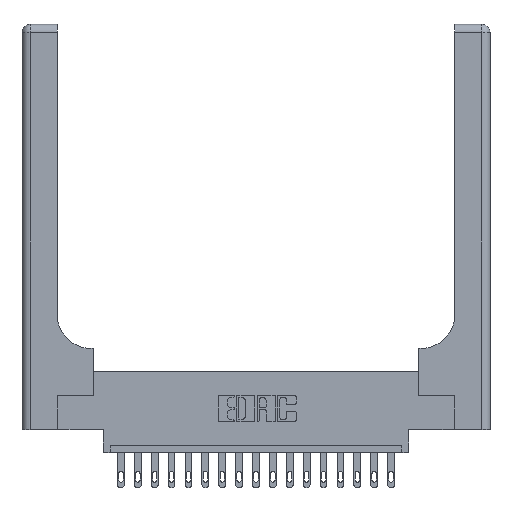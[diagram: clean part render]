
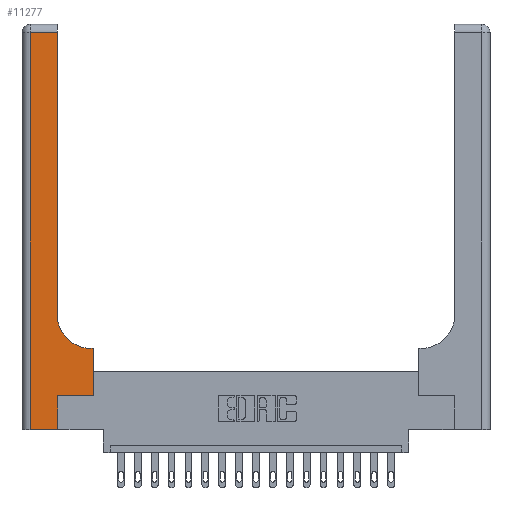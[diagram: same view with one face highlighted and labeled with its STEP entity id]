
A CAD part, top view. The second image highlights one B-rep face of the part: STEP entity #11277.
In plain terms, the highlighted planar face has unit normal (0, 0, 1).
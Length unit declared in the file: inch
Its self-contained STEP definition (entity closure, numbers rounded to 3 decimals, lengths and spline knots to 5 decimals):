
#448 = VERTEX_POINT ( 'NONE', #10915 ) ;
#597 = LINE ( 'NONE', #6665, #10438 ) ;
#862 = DIRECTION ( 'NONE',  ( -1., 0., 0. ) ) ;
#1247 = CARTESIAN_POINT ( 'NONE',  ( 0.26, 2.94, 0.37 ) ) ;
#1666 = VECTOR ( 'NONE', #3041, 39.37008 ) ;
#1766 = VERTEX_POINT ( 'NONE', #1247 ) ;
#1850 = LINE ( 'NONE', #6346, #12595 ) ;
#1892 = EDGE_CURVE ( 'NONE', #11586, #7389, #16539, .T. ) ;
#2382 = CARTESIAN_POINT ( 'NONE',  ( 0.06, 0., 0.37 ) ) ;
#2471 = ORIENTED_EDGE ( 'NONE', *, *, #11147, .T. ) ;
#2693 = DIRECTION ( 'NONE',  ( 0., 1., 0. ) ) ;
#3041 = DIRECTION ( 'NONE',  ( 0., -1., 0. ) ) ;
#3828 = ORIENTED_EDGE ( 'NONE', *, *, #5410, .T. ) ;
#3852 = LINE ( 'NONE', #8823, #18318 ) ;
#3874 = CARTESIAN_POINT ( 'NONE',  ( 0.26, 0.6, 0.37 ) ) ;
#4307 = VERTEX_POINT ( 'NONE', #8676 ) ;
#4693 = DIRECTION ( 'NONE',  ( 0., 1., 0. ) ) ;
#5379 = LINE ( 'NONE', #3874, #12411 ) ;
#5410 = EDGE_CURVE ( 'NONE', #14057, #8418, #8841, .T. ) ;
#5472 = DIRECTION ( 'NONE',  ( -1., 0., 0. ) ) ;
#6346 = CARTESIAN_POINT ( 'NONE',  ( 0.528, 0.25, 0.37 ) ) ;
#6375 = CARTESIAN_POINT ( 'NONE',  ( 0.265, 0., 0.37 ) ) ;
#6446 = CARTESIAN_POINT ( 'NONE',  ( 0.06, 2.94, 0.37 ) ) ;
#6665 = CARTESIAN_POINT ( 'NONE',  ( 0.265, 0.25, 0.37 ) ) ;
#6925 = AXIS2_PLACEMENT_3D ( 'NONE', #7197, #11944, #10188 ) ;
#7197 = CARTESIAN_POINT ( 'NONE',  ( 0.51, 0.85, 0.37 ) ) ;
#7357 = DIRECTION ( 'NONE',  ( 0., 0., -1. ) ) ;
#7389 = VERTEX_POINT ( 'NONE', #2382 ) ;
#7577 = EDGE_CURVE ( 'NONE', #14171, #4307, #1850, .T. ) ;
#8364 = LINE ( 'NONE', #12728, #13408 ) ;
#8418 = VERTEX_POINT ( 'NONE', #10773 ) ;
#8663 = CARTESIAN_POINT ( 'NONE',  ( 0., 3., 0.37 ) ) ;
#8676 = CARTESIAN_POINT ( 'NONE',  ( 0.528, 0.6, 0.37 ) ) ;
#8744 = EDGE_CURVE ( 'NONE', #8418, #1766, #11638, .T. ) ;
#8823 = CARTESIAN_POINT ( 'NONE',  ( 0., 2.94, 0.37 ) ) ;
#8841 = CIRCLE ( 'NONE', #6925, 0.25 ) ;
#9365 = LINE ( 'NONE', #6375, #12979 ) ;
#9778 = ORIENTED_EDGE ( 'NONE', *, *, #15472, .T. ) ;
#9821 = AXIS2_PLACEMENT_3D ( 'NONE', #8663, #7357, #14606 ) ;
#9897 = EDGE_CURVE ( 'NONE', #13454, #14171, #597, .T. ) ;
#10188 = DIRECTION ( 'NONE',  ( 1., 0., 0. ) ) ;
#10438 = VECTOR ( 'NONE', #12729, 39.37008 ) ;
#10483 = ORIENTED_EDGE ( 'NONE', *, *, #10532, .T. ) ;
#10532 = EDGE_CURVE ( 'NONE', #1766, #11586, #3852, .T. ) ;
#10773 = CARTESIAN_POINT ( 'NONE',  ( 0.26, 0.85, 0.37 ) ) ;
#10915 = CARTESIAN_POINT ( 'NONE',  ( 0.265, 0., 0.37 ) ) ;
#11147 = EDGE_CURVE ( 'NONE', #448, #13454, #9365, .T. ) ;
#11277 = ADVANCED_FACE ( 'NONE', ( #13415 ), #19052, .F. ) ;
#11418 = ORIENTED_EDGE ( 'NONE', *, *, #1892, .T. ) ;
#11422 = CARTESIAN_POINT ( 'NONE',  ( 0.51, 0.6, 0.37 ) ) ;
#11586 = VERTEX_POINT ( 'NONE', #6446 ) ;
#11638 = LINE ( 'NONE', #11737, #17058 ) ;
#11737 = CARTESIAN_POINT ( 'NONE',  ( 0.26, 3., 0.37 ) ) ;
#11944 = DIRECTION ( 'NONE',  ( 0., 0., -1. ) ) ;
#12411 = VECTOR ( 'NONE', #5472, 39.37008 ) ;
#12487 = ORIENTED_EDGE ( 'NONE', *, *, #14084, .T. ) ;
#12595 = VECTOR ( 'NONE', #17246, 39.37008 ) ;
#12680 = ORIENTED_EDGE ( 'NONE', *, *, #7577, .T. ) ;
#12728 = CARTESIAN_POINT ( 'NONE',  ( 0., 0., 0.37 ) ) ;
#12729 = DIRECTION ( 'NONE',  ( 1., 0., 0. ) ) ;
#12842 = ORIENTED_EDGE ( 'NONE', *, *, #8744, .T. ) ;
#12979 = VECTOR ( 'NONE', #4693, 39.37008 ) ;
#13112 = CARTESIAN_POINT ( 'NONE',  ( 0.528, 0.25, 0.37 ) ) ;
#13408 = VECTOR ( 'NONE', #15986, 39.37008 ) ;
#13415 = FACE_OUTER_BOUND ( 'NONE', #16991, .T. ) ;
#13454 = VERTEX_POINT ( 'NONE', #16218 ) ;
#14057 = VERTEX_POINT ( 'NONE', #11422 ) ;
#14084 = EDGE_CURVE ( 'NONE', #4307, #14057, #5379, .T. ) ;
#14171 = VERTEX_POINT ( 'NONE', #13112 ) ;
#14606 = DIRECTION ( 'NONE',  ( -1., 0., 0. ) ) ;
#14954 = CARTESIAN_POINT ( 'NONE',  ( 0.06, 3., 0.37 ) ) ;
#15472 = EDGE_CURVE ( 'NONE', #7389, #448, #8364, .T. ) ;
#15986 = DIRECTION ( 'NONE',  ( 1., 0., 0. ) ) ;
#16218 = CARTESIAN_POINT ( 'NONE',  ( 0.265, 0.25, 0.37 ) ) ;
#16539 = LINE ( 'NONE', #14954, #1666 ) ;
#16991 = EDGE_LOOP ( 'NONE', ( #12842, #10483, #11418, #9778, #2471, #17073, #12680, #12487, #3828 ) ) ;
#17058 = VECTOR ( 'NONE', #2693, 39.37008 ) ;
#17073 = ORIENTED_EDGE ( 'NONE', *, *, #9897, .T. ) ;
#17246 = DIRECTION ( 'NONE',  ( 0., 1., 0. ) ) ;
#18318 = VECTOR ( 'NONE', #862, 39.37008 ) ;
#19052 = PLANE ( 'NONE',  #9821 ) ;
